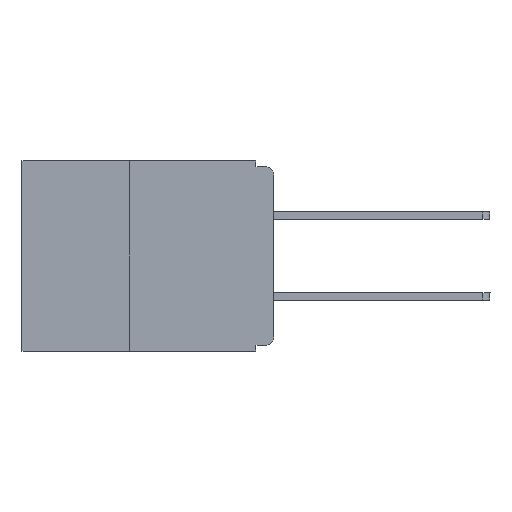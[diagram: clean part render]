
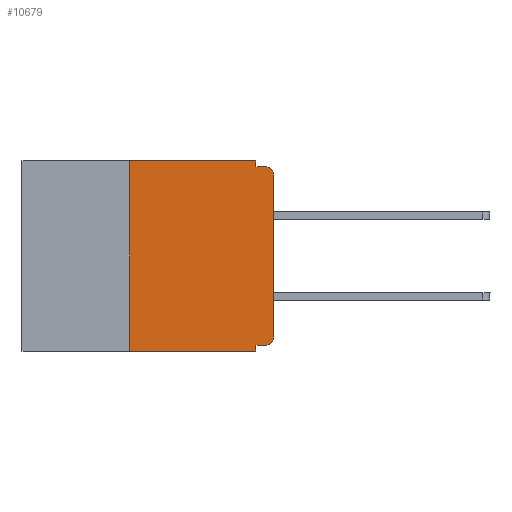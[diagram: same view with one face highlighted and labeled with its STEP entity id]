
A CAD part, left-side view. The second image highlights one B-rep face of the part: STEP entity #10679.
In plain terms, the highlighted planar face has unit normal (-1, 0, 0).
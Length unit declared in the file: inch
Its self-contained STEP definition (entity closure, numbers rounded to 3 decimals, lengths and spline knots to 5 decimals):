
#44 = VERTEX_POINT ( 'NONE', #4748 ) ;
#98 = VERTEX_POINT ( 'NONE', #4991 ) ;
#278 = EDGE_CURVE ( 'NONE', #4718, #8203, #8943, .T. ) ;
#411 = VERTEX_POINT ( 'NONE', #9964 ) ;
#474 = ORIENTED_EDGE ( 'NONE', *, *, #10599, .T. ) ;
#616 = LINE ( 'NONE', #11581, #753 ) ;
#753 = VECTOR ( 'NONE', #6879, 39.37008 ) ;
#821 = EDGE_CURVE ( 'NONE', #2464, #6251, #2184, .T. ) ;
#846 = CIRCLE ( 'NONE', #8715, 0.015 ) ;
#999 = VECTOR ( 'NONE', #5302, 39.37008 ) ;
#1057 = EDGE_CURVE ( 'NONE', #8203, #2476, #5687, .T. ) ;
#1129 = DIRECTION ( 'NONE',  ( 0., 0., -1. ) ) ;
#1388 = CARTESIAN_POINT ( 'NONE',  ( 0., 0.031, 0. ) ) ;
#1563 = DIRECTION ( 'NONE',  ( 0., 1., 0. ) ) ;
#2125 = LINE ( 'NONE', #3473, #5494 ) ;
#2184 = LINE ( 'NONE', #3445, #999 ) ;
#2199 = LINE ( 'NONE', #3261, #4104 ) ;
#2464 = VERTEX_POINT ( 'NONE', #4605 ) ;
#2476 = VERTEX_POINT ( 'NONE', #2814 ) ;
#2774 = EDGE_CURVE ( 'NONE', #44, #2464, #2125, .T. ) ;
#2810 = VERTEX_POINT ( 'NONE', #6192 ) ;
#2814 = CARTESIAN_POINT ( 'NONE',  ( 0., 0.015, -0.01 ) ) ;
#3147 = VERTEX_POINT ( 'NONE', #10421 ) ;
#3206 = PLANE ( 'NONE',  #8299 ) ;
#3261 = CARTESIAN_POINT ( 'NONE',  ( 0., 0.25, -0.33 ) ) ;
#3445 = CARTESIAN_POINT ( 'NONE',  ( 0., 0.031, -0.33 ) ) ;
#3473 = CARTESIAN_POINT ( 'NONE',  ( 0., 0., -0.32 ) ) ;
#3498 = VECTOR ( 'NONE', #7938, 39.37008 ) ;
#3507 = ORIENTED_EDGE ( 'NONE', *, *, #4984, .T. ) ;
#3916 = CARTESIAN_POINT ( 'NONE',  ( 0., 0., -0.01 ) ) ;
#3984 = EDGE_CURVE ( 'NONE', #3147, #4718, #4289, .T. ) ;
#4087 = DIRECTION ( 'NONE',  ( 0., 0., -1. ) ) ;
#4104 = VECTOR ( 'NONE', #9856, 39.37008 ) ;
#4124 = CARTESIAN_POINT ( 'NONE',  ( 0., 0.437, 0. ) ) ;
#4277 = ORIENTED_EDGE ( 'NONE', *, *, #1057, .F. ) ;
#4289 = LINE ( 'NONE', #5468, #6634 ) ;
#4409 = EDGE_CURVE ( 'NONE', #2810, #98, #616, .T. ) ;
#4605 = CARTESIAN_POINT ( 'NONE',  ( 0., 0.031, -0.32 ) ) ;
#4718 = VERTEX_POINT ( 'NONE', #11217 ) ;
#4719 = DIRECTION ( 'NONE',  ( 0., -1., 0. ) ) ;
#4748 = CARTESIAN_POINT ( 'NONE',  ( 0., 0.015, -0.32 ) ) ;
#4792 = CARTESIAN_POINT ( 'NONE',  ( 0., 0.031, -0.01 ) ) ;
#4806 = ORIENTED_EDGE ( 'NONE', *, *, #4409, .T. ) ;
#4869 = DIRECTION ( 'NONE',  ( -1., 0., 0. ) ) ;
#4984 = EDGE_CURVE ( 'NONE', #98, #2476, #6760, .T. ) ;
#4991 = CARTESIAN_POINT ( 'NONE',  ( 0., 0., -0.025 ) ) ;
#5302 = DIRECTION ( 'NONE',  ( 0., 0., -1. ) ) ;
#5385 = ORIENTED_EDGE ( 'NONE', *, *, #821, .F. ) ;
#5468 = CARTESIAN_POINT ( 'NONE',  ( 0., 0.437, 0. ) ) ;
#5494 = VECTOR ( 'NONE', #1563, 39.37008 ) ;
#5687 = LINE ( 'NONE', #3916, #5982 ) ;
#5982 = VECTOR ( 'NONE', #4719, 39.37008 ) ;
#6142 = ORIENTED_EDGE ( 'NONE', *, *, #3984, .F. ) ;
#6192 = CARTESIAN_POINT ( 'NONE',  ( 0., 0., -0.305 ) ) ;
#6251 = VERTEX_POINT ( 'NONE', #11288 ) ;
#6506 = EDGE_CURVE ( 'NONE', #411, #3147, #2199, .T. ) ;
#6634 = VECTOR ( 'NONE', #9280, 39.37008 ) ;
#6760 = CIRCLE ( 'NONE', #6990, 0.015 ) ;
#6864 = CARTESIAN_POINT ( 'NONE',  ( 0., 0.015, -0.025 ) ) ;
#6879 = DIRECTION ( 'NONE',  ( 0., 0., 1. ) ) ;
#6942 = DIRECTION ( 'NONE',  ( 0., 0., -1. ) ) ;
#6990 = AXIS2_PLACEMENT_3D ( 'NONE', #6864, #8869, #6942 ) ;
#7482 = EDGE_CURVE ( 'NONE', #411, #6251, #7882, .T. ) ;
#7585 = ORIENTED_EDGE ( 'NONE', *, *, #278, .F. ) ;
#7882 = LINE ( 'NONE', #8492, #11438 ) ;
#7938 = DIRECTION ( 'NONE',  ( 0., 0., -1. ) ) ;
#8203 = VERTEX_POINT ( 'NONE', #4792 ) ;
#8299 = AXIS2_PLACEMENT_3D ( 'NONE', #4124, #10692, #4087 ) ;
#8492 = CARTESIAN_POINT ( 'NONE',  ( 0., 0.437, -0.33 ) ) ;
#8715 = AXIS2_PLACEMENT_3D ( 'NONE', #12150, #4869, #1129 ) ;
#8869 = DIRECTION ( 'NONE',  ( -1., 0., 0. ) ) ;
#8943 = LINE ( 'NONE', #1388, #3498 ) ;
#9137 = EDGE_LOOP ( 'NONE', ( #4806, #3507, #4277, #7585, #6142, #9726, #10843, #5385, #9235, #474 ) ) ;
#9235 = ORIENTED_EDGE ( 'NONE', *, *, #2774, .F. ) ;
#9280 = DIRECTION ( 'NONE',  ( 0., -1., 0. ) ) ;
#9726 = ORIENTED_EDGE ( 'NONE', *, *, #6506, .F. ) ;
#9856 = DIRECTION ( 'NONE',  ( 0., 0., 1. ) ) ;
#9964 = CARTESIAN_POINT ( 'NONE',  ( 0., 0.25, -0.33 ) ) ;
#10308 = DIRECTION ( 'NONE',  ( 0., -1., 0. ) ) ;
#10421 = CARTESIAN_POINT ( 'NONE',  ( 0., 0.25, 0. ) ) ;
#10599 = EDGE_CURVE ( 'NONE', #44, #2810, #846, .T. ) ;
#10679 = ADVANCED_FACE ( 'NONE', ( #11752 ), #3206, .F. ) ;
#10692 = DIRECTION ( 'NONE',  ( 1., 0., 0. ) ) ;
#10843 = ORIENTED_EDGE ( 'NONE', *, *, #7482, .T. ) ;
#11217 = CARTESIAN_POINT ( 'NONE',  ( 0., 0.031, 0. ) ) ;
#11288 = CARTESIAN_POINT ( 'NONE',  ( 0., 0.031, -0.33 ) ) ;
#11438 = VECTOR ( 'NONE', #10308, 39.37008 ) ;
#11581 = CARTESIAN_POINT ( 'NONE',  ( 0., 0., 0. ) ) ;
#11752 = FACE_OUTER_BOUND ( 'NONE', #9137, .T. ) ;
#12150 = CARTESIAN_POINT ( 'NONE',  ( 0., 0.015, -0.305 ) ) ;
